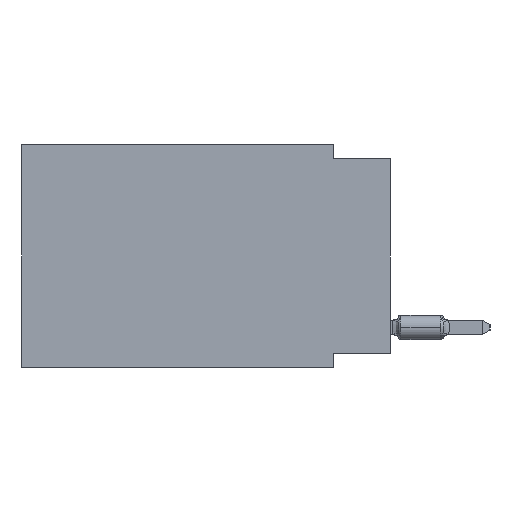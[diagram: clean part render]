
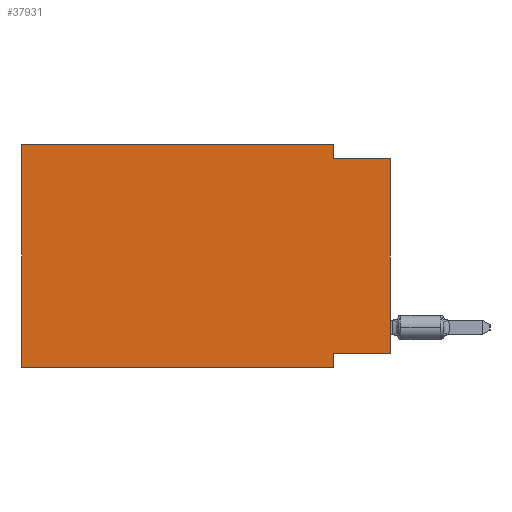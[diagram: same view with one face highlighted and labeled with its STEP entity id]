
A CAD part, left-side view. The second image highlights one B-rep face of the part: STEP entity #37931.
In plain terms, the highlighted planar face has unit normal (-1, 0, 0).
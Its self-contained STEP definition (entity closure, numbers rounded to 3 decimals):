
#1212 = CARTESIAN_POINT ( 'NONE',  ( 0., 0., -0.635 ) ) ;
#2431 = VECTOR ( 'NONE', #44765, 1000. ) ;
#2865 = CARTESIAN_POINT ( 'NONE',  ( 0., 2.54, 0. ) ) ;
#4058 = CARTESIAN_POINT ( 'NONE',  ( 0., 16.383, 0. ) ) ;
#5848 = LINE ( 'NONE', #59371, #84641 ) ;
#6341 = DIRECTION ( 'NONE',  ( 1., 0., 0. ) ) ;
#6959 = VECTOR ( 'NONE', #59324, 1000. ) ;
#7694 = DIRECTION ( 'NONE',  ( 0., 0., 1. ) ) ;
#7749 = ORIENTED_EDGE ( 'NONE', *, *, #12895, .F. ) ;
#9461 = EDGE_CURVE ( 'NONE', #14877, #50232, #5848, .T. ) ;
#9860 = LINE ( 'NONE', #2865, #77832 ) ;
#10679 = VECTOR ( 'NONE', #35422, 1000. ) ;
#11845 = VECTOR ( 'NONE', #64852, 1000. ) ;
#11857 = CARTESIAN_POINT ( 'NONE',  ( 0., 16.383, 0. ) ) ;
#12895 = EDGE_CURVE ( 'NONE', #54468, #49360, #9860, .T. ) ;
#13413 = LINE ( 'NONE', #26569, #53228 ) ;
#14877 = VERTEX_POINT ( 'NONE', #27341 ) ;
#15688 = LINE ( 'NONE', #55163, #10679 ) ;
#15944 = CARTESIAN_POINT ( 'NONE',  ( 0., 2.54, -0.635 ) ) ;
#18288 = EDGE_CURVE ( 'NONE', #72860, #54468, #33758, .T. ) ;
#19822 = EDGE_CURVE ( 'NONE', #30298, #40213, #78039, .T. ) ;
#20267 = LINE ( 'NONE', #32546, #6959 ) ;
#21955 = EDGE_CURVE ( 'NONE', #50232, #40213, #20267, .T. ) ;
#22023 = FACE_OUTER_BOUND ( 'NONE', #31827, .T. ) ;
#23161 = ORIENTED_EDGE ( 'NONE', *, *, #51331, .T. ) ;
#25445 = CARTESIAN_POINT ( 'NONE',  ( 0., 2.54, 0. ) ) ;
#26569 = CARTESIAN_POINT ( 'NONE',  ( 0., 16.383, 0. ) ) ;
#27341 = CARTESIAN_POINT ( 'NONE',  ( 0., 0., -9.271 ) ) ;
#27724 = ORIENTED_EDGE ( 'NONE', *, *, #63305, .F. ) ;
#28588 = PLANE ( 'NONE',  #63380 ) ;
#30298 = VERTEX_POINT ( 'NONE', #36228 ) ;
#31827 = EDGE_LOOP ( 'NONE', ( #23161, #27724, #7749, #62517, #44269, #74405, #46987, #74712 ) ) ;
#32041 = LINE ( 'NONE', #39049, #2431 ) ;
#32546 = CARTESIAN_POINT ( 'NONE',  ( 0., 2.54, -9.906 ) ) ;
#33758 = LINE ( 'NONE', #11857, #35355 ) ;
#35355 = VECTOR ( 'NONE', #67126, 1000. ) ;
#35422 = DIRECTION ( 'NONE',  ( 0., 0., 1. ) ) ;
#36228 = CARTESIAN_POINT ( 'NONE',  ( 0., 16.383, -9.906 ) ) ;
#37931 = ADVANCED_FACE ( 'NONE', ( #22023 ), #28588, .F. ) ;
#39049 = CARTESIAN_POINT ( 'NONE',  ( 0., 0., -0.635 ) ) ;
#40213 = VERTEX_POINT ( 'NONE', #57804 ) ;
#44269 = ORIENTED_EDGE ( 'NONE', *, *, #67300, .F. ) ;
#44765 = DIRECTION ( 'NONE',  ( 0., -1., 0. ) ) ;
#45910 = VERTEX_POINT ( 'NONE', #1212 ) ;
#46987 = ORIENTED_EDGE ( 'NONE', *, *, #21955, .F. ) ;
#49360 = VERTEX_POINT ( 'NONE', #15944 ) ;
#50203 = DIRECTION ( 'NONE',  ( 0., 0., -1. ) ) ;
#50232 = VERTEX_POINT ( 'NONE', #56101 ) ;
#51331 = EDGE_CURVE ( 'NONE', #14877, #45910, #15688, .T. ) ;
#53228 = VECTOR ( 'NONE', #7694, 1000. ) ;
#54468 = VERTEX_POINT ( 'NONE', #25445 ) ;
#55163 = CARTESIAN_POINT ( 'NONE',  ( 0., 0., 0. ) ) ;
#56101 = CARTESIAN_POINT ( 'NONE',  ( 0., 2.54, -9.271 ) ) ;
#57804 = CARTESIAN_POINT ( 'NONE',  ( 0., 2.54, -9.906 ) ) ;
#59324 = DIRECTION ( 'NONE',  ( 0., 0., -1. ) ) ;
#59371 = CARTESIAN_POINT ( 'NONE',  ( 0., 0., -9.271 ) ) ;
#62517 = ORIENTED_EDGE ( 'NONE', *, *, #18288, .F. ) ;
#63305 = EDGE_CURVE ( 'NONE', #49360, #45910, #32041, .T. ) ;
#63380 = AXIS2_PLACEMENT_3D ( 'NONE', #73916, #6341, #80473 ) ;
#64852 = DIRECTION ( 'NONE',  ( 0., -1., 0. ) ) ;
#67126 = DIRECTION ( 'NONE',  ( 0., -1., 0. ) ) ;
#67300 = EDGE_CURVE ( 'NONE', #30298, #72860, #13413, .T. ) ;
#70140 = CARTESIAN_POINT ( 'NONE',  ( 0., 16.383, -9.906 ) ) ;
#72860 = VERTEX_POINT ( 'NONE', #4058 ) ;
#73916 = CARTESIAN_POINT ( 'NONE',  ( 0., 16.383, 0. ) ) ;
#74405 = ORIENTED_EDGE ( 'NONE', *, *, #19822, .T. ) ;
#74712 = ORIENTED_EDGE ( 'NONE', *, *, #9461, .F. ) ;
#77832 = VECTOR ( 'NONE', #50203, 1000. ) ;
#78039 = LINE ( 'NONE', #70140, #11845 ) ;
#80473 = DIRECTION ( 'NONE',  ( 0., 0., -1. ) ) ;
#84641 = VECTOR ( 'NONE', #86127, 1000. ) ;
#86127 = DIRECTION ( 'NONE',  ( 0., 1., 0. ) ) ;
